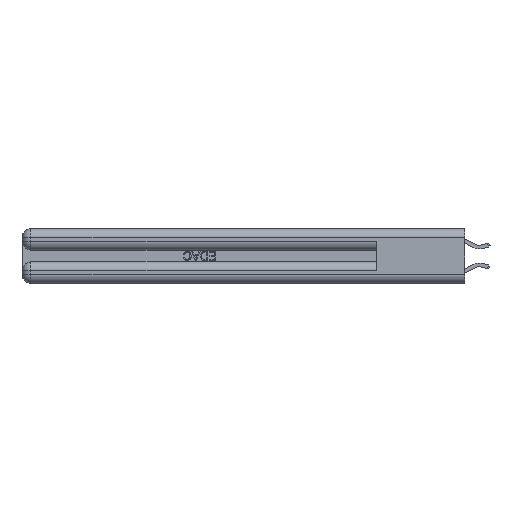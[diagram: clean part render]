
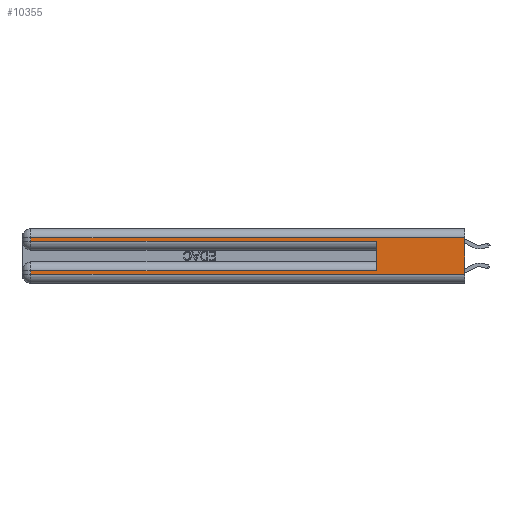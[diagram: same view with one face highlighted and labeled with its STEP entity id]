
A CAD part, left-side view. The second image highlights one B-rep face of the part: STEP entity #10355.
In plain terms, the highlighted planar face has unit normal (-1, 0, 0).
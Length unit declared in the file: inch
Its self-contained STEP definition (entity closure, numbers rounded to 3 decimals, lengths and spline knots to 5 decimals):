
#760 = VERTEX_POINT ( 'NONE', #28833 ) ;
#1366 = VERTEX_POINT ( 'NONE', #26528 ) ;
#2163 = CARTESIAN_POINT ( 'NONE',  ( 0., 2.94, 0.37 ) ) ;
#2648 = LINE ( 'NONE', #2163, #27265 ) ;
#2746 = VERTEX_POINT ( 'NONE', #11937 ) ;
#3330 = EDGE_CURVE ( 'NONE', #4158, #15855, #13919, .T. ) ;
#4080 = ORIENTED_EDGE ( 'NONE', *, *, #29457, .F. ) ;
#4158 = VERTEX_POINT ( 'NONE', #12587 ) ;
#4523 = ORIENTED_EDGE ( 'NONE', *, *, #18208, .T. ) ;
#4697 = LINE ( 'NONE', #13987, #12175 ) ;
#5135 = DIRECTION ( 'NONE',  ( 0., 0., 1. ) ) ;
#5220 = VERTEX_POINT ( 'NONE', #30408 ) ;
#6381 = ORIENTED_EDGE ( 'NONE', *, *, #11783, .T. ) ;
#6532 = EDGE_CURVE ( 'NONE', #2746, #8744, #7082, .T. ) ;
#6716 = VECTOR ( 'NONE', #24922, 39.37008 ) ;
#6738 = CARTESIAN_POINT ( 'NONE',  ( 0., 0.6, 0.145 ) ) ;
#7082 = LINE ( 'NONE', #20535, #6716 ) ;
#7695 = DIRECTION ( 'NONE',  ( 0., 0., -1. ) ) ;
#7965 = EDGE_CURVE ( 'NONE', #760, #13675, #29696, .T. ) ;
#8744 = VERTEX_POINT ( 'NONE', #25662 ) ;
#9817 = CARTESIAN_POINT ( 'NONE',  ( 0., 0., 0.085 ) ) ;
#10355 = ADVANCED_FACE ( 'NONE', ( #27529 ), #14514, .F. ) ;
#11783 = EDGE_CURVE ( 'NONE', #5220, #15855, #4697, .T. ) ;
#11937 = CARTESIAN_POINT ( 'NONE',  ( 0., 0., 0.31 ) ) ;
#12175 = VECTOR ( 'NONE', #18759, 39.37008 ) ;
#12587 = CARTESIAN_POINT ( 'NONE',  ( 0., 0.6, 0.085 ) ) ;
#12819 = VECTOR ( 'NONE', #5135, 39.37008 ) ;
#13675 = VERTEX_POINT ( 'NONE', #25873 ) ;
#13919 = LINE ( 'NONE', #6738, #12819 ) ;
#13987 = CARTESIAN_POINT ( 'NONE',  ( 0., 0., 0.285 ) ) ;
#14157 = DIRECTION ( 'NONE',  ( 0., 1., 0. ) ) ;
#14417 = DIRECTION ( 'NONE',  ( 1., 0., 0. ) ) ;
#14509 = ORIENTED_EDGE ( 'NONE', *, *, #3330, .F. ) ;
#14514 = PLANE ( 'NONE',  #29346 ) ;
#15745 = VECTOR ( 'NONE', #25503, 39.37008 ) ;
#15855 = VERTEX_POINT ( 'NONE', #25146 ) ;
#15894 = ORIENTED_EDGE ( 'NONE', *, *, #26233, .T. ) ;
#18197 = CARTESIAN_POINT ( 'NONE',  ( 0., 0., 0.06 ) ) ;
#18208 = EDGE_CURVE ( 'NONE', #13675, #1366, #21323, .T. ) ;
#18226 = VECTOR ( 'NONE', #25004, 39.37008 ) ;
#18514 = VECTOR ( 'NONE', #29000, 39.37008 ) ;
#18759 = DIRECTION ( 'NONE',  ( 0., -1., 0. ) ) ;
#19484 = CARTESIAN_POINT ( 'NONE',  ( 0., 0., 0.37 ) ) ;
#20252 = LINE ( 'NONE', #9817, #22145 ) ;
#20535 = CARTESIAN_POINT ( 'NONE',  ( 0., 0., 0.31 ) ) ;
#20885 = ORIENTED_EDGE ( 'NONE', *, *, #6532, .T. ) ;
#21323 = LINE ( 'NONE', #18197, #15745 ) ;
#22145 = VECTOR ( 'NONE', #14157, 39.37008 ) ;
#22452 = ORIENTED_EDGE ( 'NONE', *, *, #28520, .T. ) ;
#23097 = EDGE_LOOP ( 'NONE', ( #4080, #20885, #22452, #6381, #14509, #15894, #26020, #4523 ) ) ;
#24922 = DIRECTION ( 'NONE',  ( 0., 1., 0. ) ) ;
#25004 = DIRECTION ( 'NONE',  ( 0., 0., -1. ) ) ;
#25146 = CARTESIAN_POINT ( 'NONE',  ( 0., 0.6, 0.285 ) ) ;
#25503 = DIRECTION ( 'NONE',  ( 0., -1., 0. ) ) ;
#25662 = CARTESIAN_POINT ( 'NONE',  ( 0., 2.94, 0.31 ) ) ;
#25873 = CARTESIAN_POINT ( 'NONE',  ( 0., 2.94, 0.06 ) ) ;
#26020 = ORIENTED_EDGE ( 'NONE', *, *, #7965, .T. ) ;
#26233 = EDGE_CURVE ( 'NONE', #4158, #760, #20252, .T. ) ;
#26528 = CARTESIAN_POINT ( 'NONE',  ( 0., 0., 0.06 ) ) ;
#26804 = CARTESIAN_POINT ( 'NONE',  ( 0., 2.94, 0.37 ) ) ;
#27265 = VECTOR ( 'NONE', #30432, 39.37008 ) ;
#27435 = CARTESIAN_POINT ( 'NONE',  ( 0., 0., 0.37 ) ) ;
#27529 = FACE_OUTER_BOUND ( 'NONE', #23097, .T. ) ;
#28520 = EDGE_CURVE ( 'NONE', #8744, #5220, #2648, .T. ) ;
#28833 = CARTESIAN_POINT ( 'NONE',  ( 0., 2.94, 0.085 ) ) ;
#29000 = DIRECTION ( 'NONE',  ( 0., 0., -1. ) ) ;
#29346 = AXIS2_PLACEMENT_3D ( 'NONE', #19484, #14417, #7695 ) ;
#29445 = LINE ( 'NONE', #27435, #18226 ) ;
#29457 = EDGE_CURVE ( 'NONE', #2746, #1366, #29445, .T. ) ;
#29696 = LINE ( 'NONE', #26804, #18514 ) ;
#30408 = CARTESIAN_POINT ( 'NONE',  ( 0., 2.94, 0.285 ) ) ;
#30432 = DIRECTION ( 'NONE',  ( 0., 0., -1. ) ) ;
